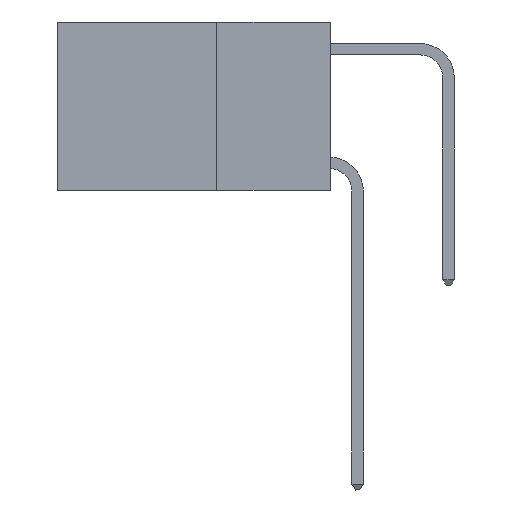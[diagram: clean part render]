
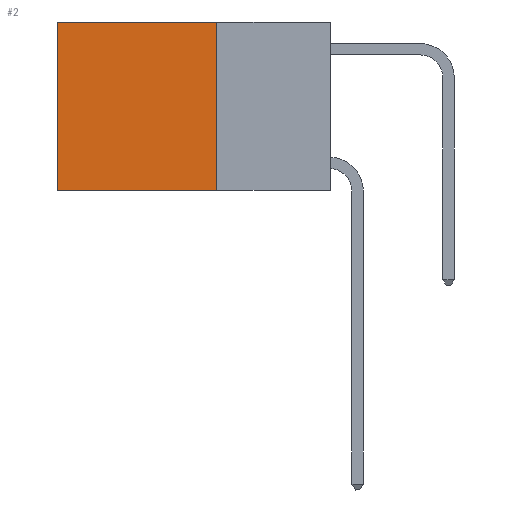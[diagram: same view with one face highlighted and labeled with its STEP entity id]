
A CAD part, left-side view. The second image highlights one B-rep face of the part: STEP entity #2.
In plain terms, the highlighted planar face has unit normal (-1, 0, 0).
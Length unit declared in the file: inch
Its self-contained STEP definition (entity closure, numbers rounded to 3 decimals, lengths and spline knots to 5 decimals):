
#2 = ADVANCED_FACE ( 'NONE', ( #812 ), #9726, .F. ) ;
#241 = EDGE_CURVE ( 'NONE', #5306, #8659, #8124, .T. ) ;
#420 = EDGE_CURVE ( 'NONE', #5306, #11484, #5524, .T. ) ;
#586 = DIRECTION ( 'NONE',  ( 1., 0., 0. ) ) ;
#812 = FACE_OUTER_BOUND ( 'NONE', #12495, .T. ) ;
#1618 = LINE ( 'NONE', #17319, #2971 ) ;
#2035 = DIRECTION ( 'NONE',  ( 0., 1., 0. ) ) ;
#2971 = VECTOR ( 'NONE', #8703, 39.37008 ) ;
#3369 = ORIENTED_EDGE ( 'NONE', *, *, #17517, .F. ) ;
#3816 = VECTOR ( 'NONE', #2035, 39.37008 ) ;
#4043 = DIRECTION ( 'NONE',  ( 0., 0., -1. ) ) ;
#4630 = CARTESIAN_POINT ( 'NONE',  ( 0.2625, 0.25, 0. ) ) ;
#5022 = ORIENTED_EDGE ( 'NONE', *, *, #420, .F. ) ;
#5306 = VERTEX_POINT ( 'NONE', #17883 ) ;
#5413 = CARTESIAN_POINT ( 'NONE',  ( 0.2625, 0.25, 0. ) ) ;
#5524 = LINE ( 'NONE', #5413, #22143 ) ;
#5977 = DIRECTION ( 'NONE',  ( 0., 1., 0. ) ) ;
#7548 = DIRECTION ( 'NONE',  ( 0., 0., -1. ) ) ;
#7765 = CARTESIAN_POINT ( 'NONE',  ( 0.2625, 0.25, 0. ) ) ;
#8124 = LINE ( 'NONE', #4630, #21793 ) ;
#8659 = VERTEX_POINT ( 'NONE', #9678 ) ;
#8703 = DIRECTION ( 'NONE',  ( 0., 0., -1. ) ) ;
#9678 = CARTESIAN_POINT ( 'NONE',  ( 0.2625, 0.6, 0. ) ) ;
#9726 = PLANE ( 'NONE',  #11523 ) ;
#11484 = VERTEX_POINT ( 'NONE', #19427 ) ;
#11523 = AXIS2_PLACEMENT_3D ( 'NONE', #7765, #586, #7548 ) ;
#12133 = CARTESIAN_POINT ( 'NONE',  ( 0.2625, 0.6, -0.37 ) ) ;
#12495 = EDGE_LOOP ( 'NONE', ( #18747, #3369, #5022, #18390 ) ) ;
#13010 = EDGE_CURVE ( 'NONE', #8659, #22286, #1618, .T. ) ;
#17319 = CARTESIAN_POINT ( 'NONE',  ( 0.2625, 0.6, 0. ) ) ;
#17517 = EDGE_CURVE ( 'NONE', #11484, #22286, #18067, .T. ) ;
#17883 = CARTESIAN_POINT ( 'NONE',  ( 0.2625, 0.25, 0. ) ) ;
#18067 = LINE ( 'NONE', #19779, #3816 ) ;
#18390 = ORIENTED_EDGE ( 'NONE', *, *, #241, .T. ) ;
#18747 = ORIENTED_EDGE ( 'NONE', *, *, #13010, .T. ) ;
#19427 = CARTESIAN_POINT ( 'NONE',  ( 0.2625, 0.25, -0.37 ) ) ;
#19779 = CARTESIAN_POINT ( 'NONE',  ( 0.2625, 0.25, -0.37 ) ) ;
#21793 = VECTOR ( 'NONE', #5977, 39.37008 ) ;
#22143 = VECTOR ( 'NONE', #4043, 39.37008 ) ;
#22286 = VERTEX_POINT ( 'NONE', #12133 ) ;
